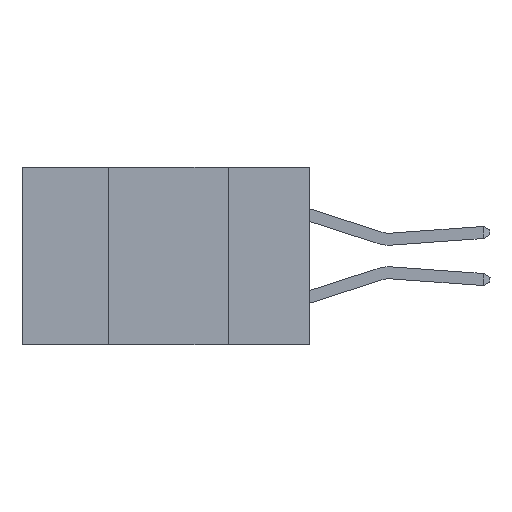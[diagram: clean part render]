
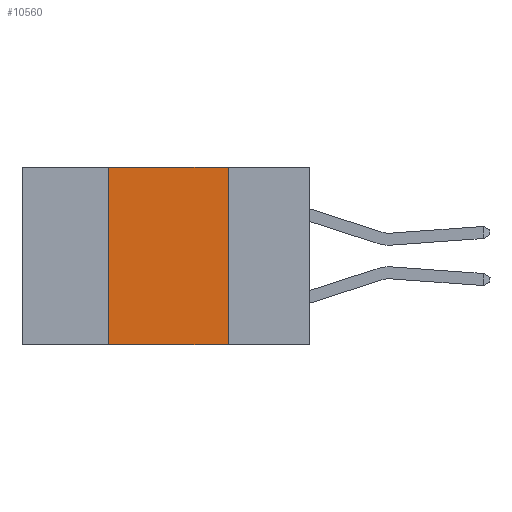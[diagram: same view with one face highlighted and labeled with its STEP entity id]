
A CAD part, left-side view. The second image highlights one B-rep face of the part: STEP entity #10560.
In plain terms, the highlighted planar face has unit normal (-1, 0, 0).
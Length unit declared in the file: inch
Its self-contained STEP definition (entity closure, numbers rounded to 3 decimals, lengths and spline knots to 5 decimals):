
#579 = EDGE_CURVE ( 'NONE', #14576, #11796, #9672, .T. ) ;
#724 = ORIENTED_EDGE ( 'NONE', *, *, #27333, .F. ) ;
#1653 = LINE ( 'NONE', #18918, #18232 ) ;
#5459 = EDGE_CURVE ( 'NONE', #14576, #19163, #13888, .T. ) ;
#5470 = CARTESIAN_POINT ( 'NONE',  ( 0., 0.6, 0. ) ) ;
#5677 = AXIS2_PLACEMENT_3D ( 'NONE', #21117, #12707, #27485 ) ;
#5935 = ORIENTED_EDGE ( 'NONE', *, *, #5459, .T. ) ;
#6646 = DIRECTION ( 'NONE',  ( 0., 0., 1. ) ) ;
#7007 = ORIENTED_EDGE ( 'NONE', *, *, #21685, .F. ) ;
#8769 = VECTOR ( 'NONE', #22549, 39.37008 ) ;
#9672 = LINE ( 'NONE', #19024, #15342 ) ;
#10560 = ADVANCED_FACE ( 'NONE', ( #14377 ), #23275, .F. ) ;
#11796 = VERTEX_POINT ( 'NONE', #23606 ) ;
#12707 = DIRECTION ( 'NONE',  ( 1., 0., 0. ) ) ;
#12817 = CARTESIAN_POINT ( 'NONE',  ( 0., 0.17, 0. ) ) ;
#13888 = LINE ( 'NONE', #18063, #24466 ) ;
#14377 = FACE_OUTER_BOUND ( 'NONE', #24146, .T. ) ;
#14576 = VERTEX_POINT ( 'NONE', #15354 ) ;
#15342 = VECTOR ( 'NONE', #6646, 39.37008 ) ;
#15354 = CARTESIAN_POINT ( 'NONE',  ( 0., 0.42, -0.37 ) ) ;
#18063 = CARTESIAN_POINT ( 'NONE',  ( 0., 0.6, -0.37 ) ) ;
#18232 = VECTOR ( 'NONE', #21022, 39.37008 ) ;
#18908 = VERTEX_POINT ( 'NONE', #12817 ) ;
#18918 = CARTESIAN_POINT ( 'NONE',  ( 0., 0.17, -0.37 ) ) ;
#19024 = CARTESIAN_POINT ( 'NONE',  ( 0., 0.42, -0.37 ) ) ;
#19163 = VERTEX_POINT ( 'NONE', #26616 ) ;
#19409 = LINE ( 'NONE', #5470, #8769 ) ;
#19642 = ORIENTED_EDGE ( 'NONE', *, *, #579, .F. ) ;
#20154 = DIRECTION ( 'NONE',  ( 0., -1., 0. ) ) ;
#21022 = DIRECTION ( 'NONE',  ( 0., 0., -1. ) ) ;
#21117 = CARTESIAN_POINT ( 'NONE',  ( 0., 0.6, 0. ) ) ;
#21685 = EDGE_CURVE ( 'NONE', #18908, #19163, #1653, .T. ) ;
#22549 = DIRECTION ( 'NONE',  ( 0., -1., 0. ) ) ;
#23275 = PLANE ( 'NONE',  #5677 ) ;
#23606 = CARTESIAN_POINT ( 'NONE',  ( 0., 0.42, 0. ) ) ;
#24146 = EDGE_LOOP ( 'NONE', ( #7007, #724, #19642, #5935 ) ) ;
#24466 = VECTOR ( 'NONE', #20154, 39.37008 ) ;
#26616 = CARTESIAN_POINT ( 'NONE',  ( 0., 0.17, -0.37 ) ) ;
#27333 = EDGE_CURVE ( 'NONE', #11796, #18908, #19409, .T. ) ;
#27485 = DIRECTION ( 'NONE',  ( 0., 0., -1. ) ) ;
